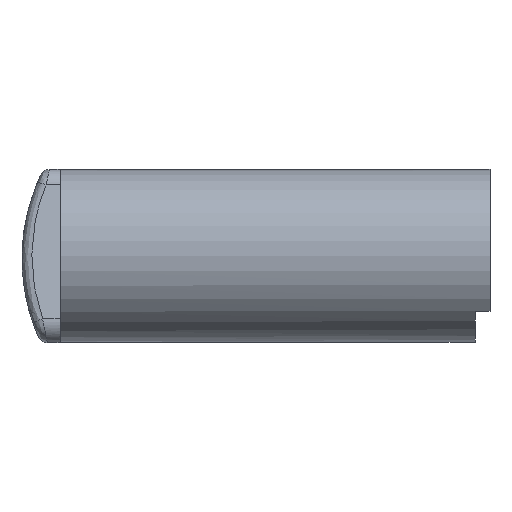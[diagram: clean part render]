
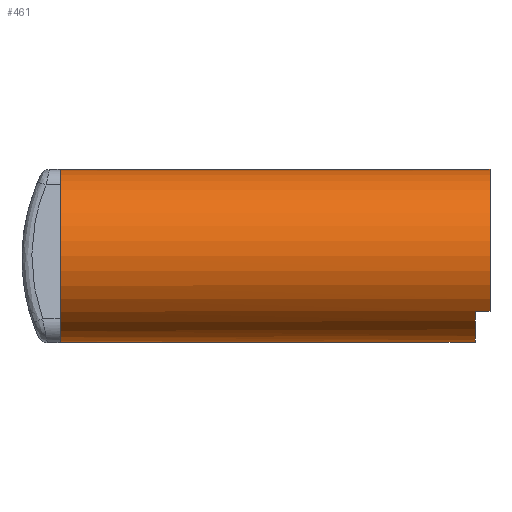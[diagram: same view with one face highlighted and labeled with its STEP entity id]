
A CAD part, front view. The second image highlights one B-rep face of the part: STEP entity #461.
In plain terms, the highlighted cylindrical face has radius 4.4 mm (diameter 8.8 mm), a full revolution.
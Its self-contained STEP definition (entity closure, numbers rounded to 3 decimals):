
#15=FACE_BOUND('',#84,.T.);
#55=FACE_OUTER_BOUND('',#83,.T.);
#83=EDGE_LOOP('',(#382,#383,#384,#385,#386,#387,#388,#389,#390,#391,#392,
#393,#394,#395));
#84=EDGE_LOOP('',(#396,#397,#398,#399));
#108=CIRCLE('',#514,4.4);
#109=CIRCLE('',#516,4.4);
#110=CIRCLE('',#517,4.4);
#111=CIRCLE('',#518,4.4);
#112=CIRCLE('',#519,4.4);
#113=CIRCLE('',#520,4.4);
#114=CIRCLE('',#521,4.4);
#115=CIRCLE('',#522,4.4);
#130=LINE('',#940,#162);
#136=LINE('',#957,#168);
#137=LINE('',#961,#169);
#138=LINE('',#965,#170);
#139=LINE('',#968,#171);
#140=LINE('',#969,#172);
#141=LINE('',#976,#173);
#142=LINE('',#979,#174);
#162=VECTOR('',#598,10.);
#168=VECTOR('',#616,10.);
#169=VECTOR('',#619,10.);
#170=VECTOR('',#622,4.4);
#171=VECTOR('',#625,10.);
#172=VECTOR('',#626,10.);
#173=VECTOR('',#633,10.);
#174=VECTOR('',#636,10.);
#181=B_SPLINE_CURVE_WITH_KNOTS('',3,(#712,#713,#714,#715,#716,#717),
 .UNSPECIFIED.,.F.,.F.,(4,1,1,4),(-0.619,-0.354,
-0.177,0.),.UNSPECIFIED.);
#194=VERTEX_POINT('',#676);
#196=VERTEX_POINT('',#710);
#217=VERTEX_POINT('',#937);
#218=VERTEX_POINT('',#939);
#221=VERTEX_POINT('',#951);
#222=VERTEX_POINT('',#955);
#223=VERTEX_POINT('',#956);
#224=VERTEX_POINT('',#958);
#225=VERTEX_POINT('',#960);
#226=VERTEX_POINT('',#962);
#227=VERTEX_POINT('',#964);
#228=VERTEX_POINT('',#966);
#229=VERTEX_POINT('',#972);
#230=VERTEX_POINT('',#973);
#231=VERTEX_POINT('',#975);
#232=VERTEX_POINT('',#977);
#238=EDGE_CURVE('',#196,#194,#181,.T.);
#273=EDGE_CURVE('',#217,#218,#130,.T.);
#279=EDGE_CURVE('',#221,#218,#108,.T.);
#281=EDGE_CURVE('',#222,#223,#136,.T.);
#282=EDGE_CURVE('',#223,#224,#109,.T.);
#283=EDGE_CURVE('',#224,#225,#137,.T.);
#284=EDGE_CURVE('',#226,#225,#110,.T.);
#285=EDGE_CURVE('',#226,#227,#138,.T.);
#286=EDGE_CURVE('',#227,#228,#111,.T.);
#287=EDGE_CURVE('',#228,#194,#139,.T.);
#288=EDGE_CURVE('',#196,#221,#140,.T.);
#289=EDGE_CURVE('',#217,#227,#112,.T.);
#290=EDGE_CURVE('',#222,#226,#113,.T.);
#291=EDGE_CURVE('',#229,#230,#114,.T.);
#292=EDGE_CURVE('',#230,#231,#141,.T.);
#293=EDGE_CURVE('',#231,#232,#115,.T.);
#294=EDGE_CURVE('',#232,#229,#142,.T.);
#382=ORIENTED_EDGE('',*,*,#281,.T.);
#383=ORIENTED_EDGE('',*,*,#282,.T.);
#384=ORIENTED_EDGE('',*,*,#283,.T.);
#385=ORIENTED_EDGE('',*,*,#284,.F.);
#386=ORIENTED_EDGE('',*,*,#285,.T.);
#387=ORIENTED_EDGE('',*,*,#286,.T.);
#388=ORIENTED_EDGE('',*,*,#287,.T.);
#389=ORIENTED_EDGE('',*,*,#238,.F.);
#390=ORIENTED_EDGE('',*,*,#288,.T.);
#391=ORIENTED_EDGE('',*,*,#279,.T.);
#392=ORIENTED_EDGE('',*,*,#273,.F.);
#393=ORIENTED_EDGE('',*,*,#289,.T.);
#394=ORIENTED_EDGE('',*,*,#285,.F.);
#395=ORIENTED_EDGE('',*,*,#290,.F.);
#396=ORIENTED_EDGE('',*,*,#291,.T.);
#397=ORIENTED_EDGE('',*,*,#292,.T.);
#398=ORIENTED_EDGE('',*,*,#293,.T.);
#399=ORIENTED_EDGE('',*,*,#294,.T.);
#442=CYLINDRICAL_SURFACE('',#515,4.4);
#461=ADVANCED_FACE('',(#55,#15),#442,.T.);
#514=AXIS2_PLACEMENT_3D('',#952,#611,#612);
#515=AXIS2_PLACEMENT_3D('',#954,#614,#615);
#516=AXIS2_PLACEMENT_3D('',#959,#617,#618);
#517=AXIS2_PLACEMENT_3D('',#963,#620,#621);
#518=AXIS2_PLACEMENT_3D('',#967,#623,#624);
#519=AXIS2_PLACEMENT_3D('',#970,#627,#628);
#520=AXIS2_PLACEMENT_3D('',#971,#629,#630);
#521=AXIS2_PLACEMENT_3D('',#974,#631,#632);
#522=AXIS2_PLACEMENT_3D('',#978,#634,#635);
#598=DIRECTION('',(1.,0.,0.));
#611=DIRECTION('center_axis',(1.,0.,0.));
#612=DIRECTION('ref_axis',(0.,1.,0.));
#614=DIRECTION('center_axis',(1.,0.,0.));
#615=DIRECTION('ref_axis',(0.,1.,0.));
#616=DIRECTION('',(-1.,0.,0.));
#617=DIRECTION('center_axis',(-1.,0.,0.));
#618=DIRECTION('ref_axis',(0.,1.,0.));
#619=DIRECTION('',(1.,0.,0.));
#620=DIRECTION('center_axis',(1.,0.,0.));
#621=DIRECTION('ref_axis',(0.,1.,0.));
#622=DIRECTION('',(-1.,0.,0.));
#623=DIRECTION('center_axis',(1.,0.,0.));
#624=DIRECTION('ref_axis',(0.,1.,0.));
#625=DIRECTION('',(-1.,0.,0.));
#626=DIRECTION('',(1.,0.,0.));
#627=DIRECTION('center_axis',(1.,0.,0.));
#628=DIRECTION('ref_axis',(0.,1.,0.));
#629=DIRECTION('center_axis',(1.,0.,0.));
#630=DIRECTION('ref_axis',(0.,1.,0.));
#631=DIRECTION('center_axis',(1.,0.,0.));
#632=DIRECTION('ref_axis',(0.,1.,0.));
#633=DIRECTION('',(-1.,0.,0.));
#634=DIRECTION('center_axis',(-1.,0.,0.));
#635=DIRECTION('ref_axis',(0.,1.,0.));
#636=DIRECTION('',(1.,0.,0.));
#676=CARTESIAN_POINT('',(-0.649,3.5,-4.4));
#710=CARTESIAN_POINT('',(-1.439,7.9,0.));
#712=CARTESIAN_POINT('Ctrl Pts',(-1.439,7.9,0.));
#713=CARTESIAN_POINT('Ctrl Pts',(-1.451,7.9,-0.998));
#714=CARTESIAN_POINT('Ctrl Pts',(-1.235,7.309,-2.638));
#715=CARTESIAN_POINT('Ctrl Pts',(-0.775,5.487,-4.087));
#716=CARTESIAN_POINT('Ctrl Pts',(-0.649,4.165,-4.4));
#717=CARTESIAN_POINT('Ctrl Pts',(-0.649,3.5,-4.4));
#937=CARTESIAN_POINT('',(0.,3.5,4.4));
#939=CARTESIAN_POINT('',(0.51,3.5,4.4));
#940=CARTESIAN_POINT('',(0.,3.5,4.4));
#951=CARTESIAN_POINT('',(0.51,7.9,0.));
#952=CARTESIAN_POINT('Origin',(0.51,3.5,0.));
#954=CARTESIAN_POINT('Origin',(0.,3.5,0.));
#955=CARTESIAN_POINT('',(21.85,6.894,-2.8));
#956=CARTESIAN_POINT('',(21.1,6.894,-2.8));
#957=CARTESIAN_POINT('',(0.,6.894,-2.8));
#958=CARTESIAN_POINT('',(21.1,0.106,-2.8));
#959=CARTESIAN_POINT('Origin',(21.1,3.5,0.));
#960=CARTESIAN_POINT('',(21.85,0.106,-2.8));
#961=CARTESIAN_POINT('',(0.,0.106,-2.8));
#962=CARTESIAN_POINT('',(21.85,-0.9,0.));
#963=CARTESIAN_POINT('Origin',(21.85,3.5,0.));
#964=CARTESIAN_POINT('',(0.,-0.9,0.));
#965=CARTESIAN_POINT('',(0.,-0.9,0.));
#966=CARTESIAN_POINT('',(0.,3.5,-4.4));
#967=CARTESIAN_POINT('Origin',(0.,3.5,0.));
#968=CARTESIAN_POINT('',(0.,3.5,-4.4));
#969=CARTESIAN_POINT('',(0.,7.9,0.));
#970=CARTESIAN_POINT('Origin',(0.,3.5,0.));
#971=CARTESIAN_POINT('Origin',(21.85,3.5,0.));
#972=CARTESIAN_POINT('',(19.15,3.85,-4.386));
#973=CARTESIAN_POINT('',(19.15,3.85,4.386));
#974=CARTESIAN_POINT('Origin',(19.15,3.5,0.));
#975=CARTESIAN_POINT('',(7.65,3.85,4.386));
#976=CARTESIAN_POINT('',(0.,3.85,4.386));
#977=CARTESIAN_POINT('',(7.65,3.85,-4.386));
#978=CARTESIAN_POINT('Origin',(7.65,3.5,0.));
#979=CARTESIAN_POINT('',(0.,3.85,-4.386));
